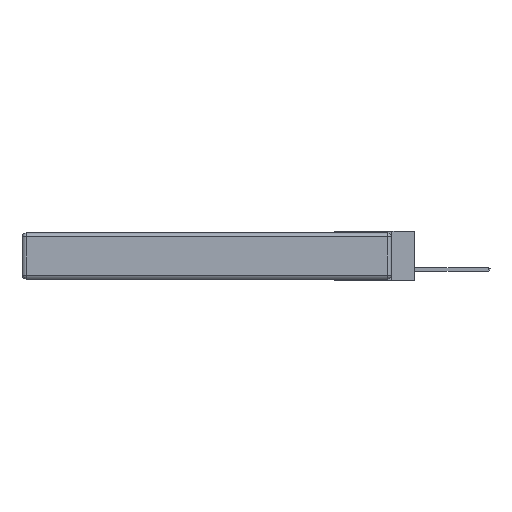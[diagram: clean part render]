
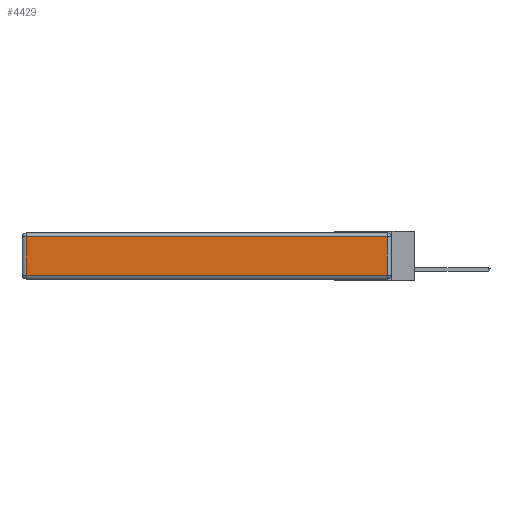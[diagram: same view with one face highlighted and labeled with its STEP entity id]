
A CAD part, left-side view. The second image highlights one B-rep face of the part: STEP entity #4429.
In plain terms, the highlighted planar face has unit normal (-1, 0, 0).
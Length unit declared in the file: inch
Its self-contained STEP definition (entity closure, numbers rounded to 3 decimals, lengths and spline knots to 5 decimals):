
#110 = ORIENTED_EDGE ( 'NONE', *, *, #13327, .T. ) ;
#171 = CARTESIAN_POINT ( 'NONE',  ( 0., 2.75, -0.03 ) ) ;
#212 = CARTESIAN_POINT ( 'NONE',  ( 0., 0., -0.313 ) ) ;
#651 = EDGE_CURVE ( 'NONE', #3468, #4063, #10150, .T. ) ;
#718 = LINE ( 'NONE', #5666, #3582 ) ;
#1392 = VECTOR ( 'NONE', #2155, 39.37008 ) ;
#1530 = FACE_OUTER_BOUND ( 'NONE', #5012, .T. ) ;
#1611 = DIRECTION ( 'NONE',  ( 0., 0., -1. ) ) ;
#1624 = CARTESIAN_POINT ( 'NONE',  ( 0., 0.03, -0.313 ) ) ;
#1918 = DIRECTION ( 'NONE',  ( 0., 0., 1. ) ) ;
#2155 = DIRECTION ( 'NONE',  ( 0., 1., 0. ) ) ;
#2193 = CARTESIAN_POINT ( 'NONE',  ( 0., 2.72, -0.03 ) ) ;
#2756 = ORIENTED_EDGE ( 'NONE', *, *, #10134, .T. ) ;
#3314 = CARTESIAN_POINT ( 'NONE',  ( 0., 0.03, -0.343 ) ) ;
#3331 = VERTEX_POINT ( 'NONE', #2193 ) ;
#3387 = EDGE_CURVE ( 'NONE', #3331, #13032, #718, .T. ) ;
#3400 = ORIENTED_EDGE ( 'NONE', *, *, #651, .T. ) ;
#3468 = VERTEX_POINT ( 'NONE', #1624 ) ;
#3582 = VECTOR ( 'NONE', #1611, 39.37008 ) ;
#3694 = ORIENTED_EDGE ( 'NONE', *, *, #3387, .T. ) ;
#4063 = VERTEX_POINT ( 'NONE', #7052 ) ;
#4429 = ADVANCED_FACE ( 'NONE', ( #1530 ), #13812, .T. ) ;
#5012 = EDGE_LOOP ( 'NONE', ( #2756, #3400, #110, #3694 ) ) ;
#5666 = CARTESIAN_POINT ( 'NONE',  ( 0., 2.72, -0.343 ) ) ;
#5950 = CARTESIAN_POINT ( 'NONE',  ( 0., 2.72, -0.313 ) ) ;
#7052 = CARTESIAN_POINT ( 'NONE',  ( 0., 0.03, -0.03 ) ) ;
#7675 = DIRECTION ( 'NONE',  ( 0., -1., 0. ) ) ;
#8397 = LINE ( 'NONE', #171, #1392 ) ;
#9521 = CARTESIAN_POINT ( 'NONE',  ( 0., 0., -0.343 ) ) ;
#9579 = DIRECTION ( 'NONE',  ( -1., 0., 0. ) ) ;
#9838 = VECTOR ( 'NONE', #12940, 39.37008 ) ;
#10134 = EDGE_CURVE ( 'NONE', #13032, #3468, #11474, .T. ) ;
#10150 = LINE ( 'NONE', #3314, #9838 ) ;
#10794 = AXIS2_PLACEMENT_3D ( 'NONE', #9521, #9579, #1918 ) ;
#11474 = LINE ( 'NONE', #212, #11989 ) ;
#11989 = VECTOR ( 'NONE', #7675, 39.37008 ) ;
#12940 = DIRECTION ( 'NONE',  ( 0., 0., 1. ) ) ;
#13032 = VERTEX_POINT ( 'NONE', #5950 ) ;
#13327 = EDGE_CURVE ( 'NONE', #4063, #3331, #8397, .T. ) ;
#13812 = PLANE ( 'NONE',  #10794 ) ;
